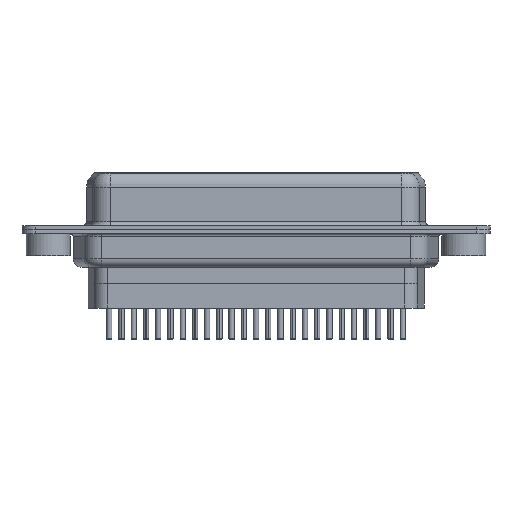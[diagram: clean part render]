
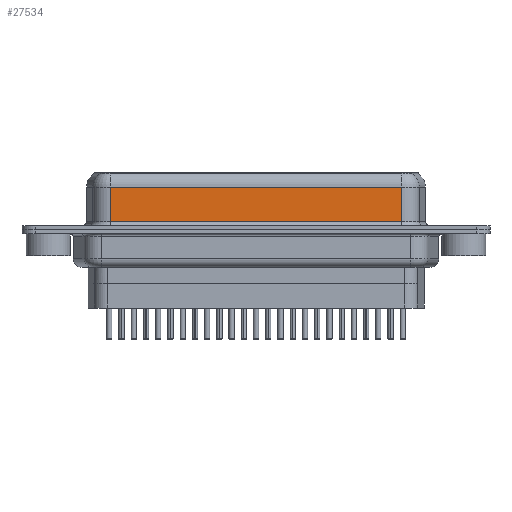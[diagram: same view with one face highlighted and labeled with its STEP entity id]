
A CAD part, front view. The second image highlights one B-rep face of the part: STEP entity #27534.
In plain terms, the highlighted planar face has unit normal (0, -1, 0).
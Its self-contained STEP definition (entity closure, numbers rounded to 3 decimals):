
#2071 = VECTOR ( 'NONE', #6048, 1000. ) ;
#2338 = ORIENTED_EDGE ( 'NONE', *, *, #27464, .F. ) ;
#3106 = DIRECTION ( 'NONE',  ( 1., 0., 0. ) ) ;
#3286 = LINE ( 'NONE', #17625, #2071 ) ;
#3827 = EDGE_CURVE ( 'NONE', #21032, #4400, #23979, .T. ) ;
#4025 = CARTESIAN_POINT ( 'NONE',  ( 40.032, -3.95, 6.6 ) ) ;
#4400 = VERTEX_POINT ( 'NONE', #13282 ) ;
#4745 = CARTESIAN_POINT ( 'NONE',  ( 40.032, -3.95, 4.85 ) ) ;
#5545 = CARTESIAN_POINT ( 'NONE',  ( 40.032, -3.95, 0.95 ) ) ;
#6048 = DIRECTION ( 'NONE',  ( -1., 0., 0. ) ) ;
#6461 = FACE_OUTER_BOUND ( 'NONE', #26379, .T. ) ;
#8151 = EDGE_CURVE ( 'NONE', #10142, #21032, #12488, .T. ) ;
#8597 = DIRECTION ( 'NONE',  ( 0., 0., -1. ) ) ;
#10142 = VERTEX_POINT ( 'NONE', #18877 ) ;
#10356 = CARTESIAN_POINT ( 'NONE',  ( 7.008, -3.95, 6.6 ) ) ;
#10440 = VECTOR ( 'NONE', #19651, 1000. ) ;
#11859 = ORIENTED_EDGE ( 'NONE', *, *, #3827, .T. ) ;
#12488 = LINE ( 'NONE', #10356, #10440 ) ;
#13282 = CARTESIAN_POINT ( 'NONE',  ( 40.032, -3.95, 0.95 ) ) ;
#14679 = VECTOR ( 'NONE', #8597, 1000. ) ;
#15766 = DIRECTION ( 'NONE',  ( 0., 1., 0. ) ) ;
#17219 = CARTESIAN_POINT ( 'NONE',  ( 7.008, -3.95, 0.95 ) ) ;
#17625 = CARTESIAN_POINT ( 'NONE',  ( 40.032, -3.95, 4.85 ) ) ;
#17822 = VECTOR ( 'NONE', #3106, 1000. ) ;
#18877 = CARTESIAN_POINT ( 'NONE',  ( 7.008, -3.95, 4.85 ) ) ;
#19651 = DIRECTION ( 'NONE',  ( 0., 0., -1. ) ) ;
#21032 = VERTEX_POINT ( 'NONE', #17219 ) ;
#22242 = VERTEX_POINT ( 'NONE', #4745 ) ;
#23979 = LINE ( 'NONE', #5545, #17822 ) ;
#24275 = ORIENTED_EDGE ( 'NONE', *, *, #8151, .T. ) ;
#25048 = DIRECTION ( 'NONE',  ( 0., 0., 1. ) ) ;
#25197 = LINE ( 'NONE', #4025, #14679 ) ;
#25407 = AXIS2_PLACEMENT_3D ( 'NONE', #27206, #15766, #25048 ) ;
#26379 = EDGE_LOOP ( 'NONE', ( #2338, #28328, #24275, #11859 ) ) ;
#27206 = CARTESIAN_POINT ( 'NONE',  ( 40.032, -3.95, 6.6 ) ) ;
#27464 = EDGE_CURVE ( 'NONE', #22242, #4400, #25197, .T. ) ;
#27534 = ADVANCED_FACE ( 'NONE', ( #6461 ), #29939, .F. ) ;
#28060 = EDGE_CURVE ( 'NONE', #22242, #10142, #3286, .T. ) ;
#28328 = ORIENTED_EDGE ( 'NONE', *, *, #28060, .T. ) ;
#29939 = PLANE ( 'NONE',  #25407 ) ;
